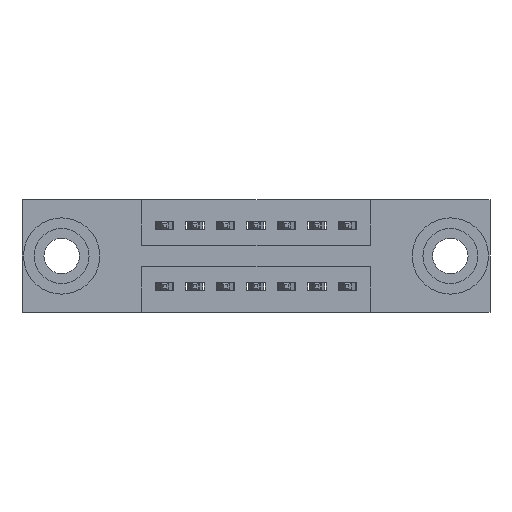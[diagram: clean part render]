
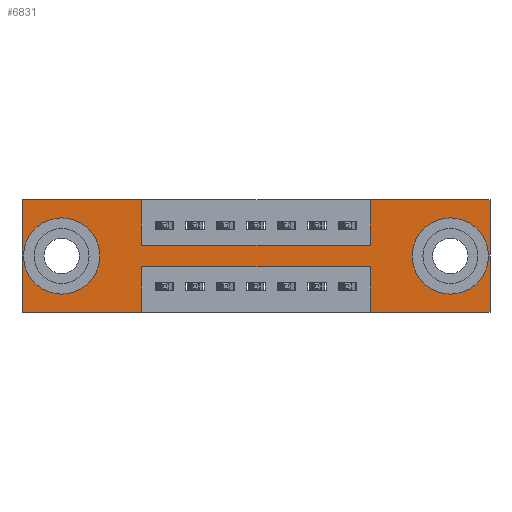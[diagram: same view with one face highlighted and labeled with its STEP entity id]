
A CAD part, front view. The second image highlights one B-rep face of the part: STEP entity #6831.
In plain terms, the highlighted planar face has unit normal (0, -1, 0).
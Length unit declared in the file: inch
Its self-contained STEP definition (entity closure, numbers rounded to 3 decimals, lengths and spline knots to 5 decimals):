
#35 = DIRECTION ( 'NONE',  ( 1., 0., 0. ) ) ;
#153 = CIRCLE ( 'NONE', #6250, 0.078 ) ;
#190 = ORIENTED_EDGE ( 'NONE', *, *, #2912, .T. ) ;
#196 = VERTEX_POINT ( 'NONE', #5397 ) ;
#292 = DIRECTION ( 'NONE',  ( 0., 0., 1. ) ) ;
#322 = ORIENTED_EDGE ( 'NONE', *, *, #9710, .F. ) ;
#339 = ORIENTED_EDGE ( 'NONE', *, *, #6166, .F. ) ;
#712 = LINE ( 'NONE', #8109, #2543 ) ;
#912 = EDGE_LOOP ( 'NONE', ( #339, #1281, #2503, #10819, #2200, #2642, #5281, #9050, #322, #3176, #4669, #4820 ) ) ;
#993 = VECTOR ( 'NONE', #8894, 39.37008 ) ;
#1029 = DIRECTION ( 'NONE',  ( 0., 1., 0. ) ) ;
#1041 = CARTESIAN_POINT ( 'NONE',  ( 1.405, 0., -0.107 ) ) ;
#1169 = DIRECTION ( 'NONE',  ( 0., 1., 0. ) ) ;
#1196 = DIRECTION ( 'NONE',  ( 0., -1., 0. ) ) ;
#1241 = DIRECTION ( 'NONE',  ( -1., 0., 0. ) ) ;
#1276 = CARTESIAN_POINT ( 'NONE',  ( 0., 0., 0. ) ) ;
#1281 = ORIENTED_EDGE ( 'NONE', *, *, #8150, .F. ) ;
#1425 = CARTESIAN_POINT ( 'NONE',  ( 0., 0., 0. ) ) ;
#1426 = CARTESIAN_POINT ( 'NONE',  ( 0.13, 0., -0.107 ) ) ;
#1484 = CARTESIAN_POINT ( 'NONE',  ( 1.1425, 0., -0.15 ) ) ;
#1490 = VECTOR ( 'NONE', #9265, 39.37008 ) ;
#1524 = CARTESIAN_POINT ( 'NONE',  ( 1.535, 0., 0. ) ) ;
#1543 = VECTOR ( 'NONE', #2429, 39.37008 ) ;
#1681 = DIRECTION ( 'NONE',  ( 0., 0., -1. ) ) ;
#1714 = DIRECTION ( 'NONE',  ( 0., 1., 0. ) ) ;
#1771 = LINE ( 'NONE', #2597, #1490 ) ;
#1783 = CARTESIAN_POINT ( 'NONE',  ( 1.405, 0., -0.185 ) ) ;
#1834 = VECTOR ( 'NONE', #7708, 39.37008 ) ;
#1903 = ORIENTED_EDGE ( 'NONE', *, *, #5004, .T. ) ;
#1976 = CARTESIAN_POINT ( 'NONE',  ( 0.13, 0., -0.263 ) ) ;
#2084 = FACE_BOUND ( 'NONE', #3840, .T. ) ;
#2121 = VERTEX_POINT ( 'NONE', #4787 ) ;
#2133 = CARTESIAN_POINT ( 'NONE',  ( 0., 0., -0.37 ) ) ;
#2169 = LINE ( 'NONE', #1425, #6464 ) ;
#2200 = ORIENTED_EDGE ( 'NONE', *, *, #6465, .F. ) ;
#2245 = VECTOR ( 'NONE', #5411, 39.37008 ) ;
#2429 = DIRECTION ( 'NONE',  ( 0., 0., -1. ) ) ;
#2431 = VERTEX_POINT ( 'NONE', #1426 ) ;
#2474 = VERTEX_POINT ( 'NONE', #10308 ) ;
#2503 = ORIENTED_EDGE ( 'NONE', *, *, #5922, .F. ) ;
#2543 = VECTOR ( 'NONE', #3100, 39.37008 ) ;
#2597 = CARTESIAN_POINT ( 'NONE',  ( 0.3925, 0., 0. ) ) ;
#2642 = ORIENTED_EDGE ( 'NONE', *, *, #5059, .F. ) ;
#2845 = LINE ( 'NONE', #5032, #5088 ) ;
#2912 = EDGE_CURVE ( 'NONE', #6247, #6154, #6344, .T. ) ;
#3100 = DIRECTION ( 'NONE',  ( 1., 0., 0. ) ) ;
#3105 = EDGE_CURVE ( 'NONE', #8250, #6004, #2169, .T. ) ;
#3176 = ORIENTED_EDGE ( 'NONE', *, *, #3105, .F. ) ;
#3223 = LINE ( 'NONE', #7791, #9541 ) ;
#3261 = VECTOR ( 'NONE', #9844, 39.37008 ) ;
#3314 = CARTESIAN_POINT ( 'NONE',  ( 1.1425, 0., -0.37 ) ) ;
#3840 = EDGE_LOOP ( 'NONE', ( #8541, #190 ) ) ;
#3850 = ORIENTED_EDGE ( 'NONE', *, *, #4265, .T. ) ;
#3860 = VECTOR ( 'NONE', #1241, 39.37008 ) ;
#4164 = CARTESIAN_POINT ( 'NONE',  ( 0.3925, 0., -0.15 ) ) ;
#4219 = EDGE_CURVE ( 'NONE', #5334, #4577, #2845, .T. ) ;
#4265 = EDGE_CURVE ( 'NONE', #8760, #2431, #153, .T. ) ;
#4519 = EDGE_CURVE ( 'NONE', #196, #8250, #7235, .T. ) ;
#4528 = LINE ( 'NONE', #4578, #9403 ) ;
#4534 = VERTEX_POINT ( 'NONE', #1484 ) ;
#4577 = VERTEX_POINT ( 'NONE', #3314 ) ;
#4578 = CARTESIAN_POINT ( 'NONE',  ( 0.3925, 0., -0.22 ) ) ;
#4655 = FACE_OUTER_BOUND ( 'NONE', #912, .T. ) ;
#4669 = ORIENTED_EDGE ( 'NONE', *, *, #4519, .F. ) ;
#4693 = CARTESIAN_POINT ( 'NONE',  ( 0.3925, 0., -0.22 ) ) ;
#4712 = CARTESIAN_POINT ( 'NONE',  ( 1.405, 0., -0.263 ) ) ;
#4787 = CARTESIAN_POINT ( 'NONE',  ( 1.535, 0., 0. ) ) ;
#4803 = LINE ( 'NONE', #6277, #2245 ) ;
#4820 = ORIENTED_EDGE ( 'NONE', *, *, #8890, .F. ) ;
#4956 = CIRCLE ( 'NONE', #7176, 0.078 ) ;
#5004 = EDGE_CURVE ( 'NONE', #2431, #8760, #4956, .T. ) ;
#5032 = CARTESIAN_POINT ( 'NONE',  ( 0., 0., -0.37 ) ) ;
#5059 = EDGE_CURVE ( 'NONE', #5090, #2121, #5572, .T. ) ;
#5088 = VECTOR ( 'NONE', #7942, 39.37008 ) ;
#5090 = VERTEX_POINT ( 'NONE', #9714 ) ;
#5281 = ORIENTED_EDGE ( 'NONE', *, *, #7440, .F. ) ;
#5296 = AXIS2_PLACEMENT_3D ( 'NONE', #6232, #1029, #7084 ) ;
#5334 = VERTEX_POINT ( 'NONE', #7845 ) ;
#5379 = DIRECTION ( 'NONE',  ( -1., 0., 0. ) ) ;
#5391 = CIRCLE ( 'NONE', #5296, 0.078 ) ;
#5397 = CARTESIAN_POINT ( 'NONE',  ( 0., 0., -0.37 ) ) ;
#5411 = DIRECTION ( 'NONE',  ( 0., 0., -1. ) ) ;
#5503 = DIRECTION ( 'NONE',  ( 0., 1., 0. ) ) ;
#5572 = LINE ( 'NONE', #1276, #993 ) ;
#5612 = EDGE_CURVE ( 'NONE', #8415, #4534, #712, .T. ) ;
#5922 = EDGE_CURVE ( 'NONE', #4577, #9687, #6406, .T. ) ;
#6004 = VERTEX_POINT ( 'NONE', #7778 ) ;
#6134 = LINE ( 'NONE', #1524, #1543 ) ;
#6154 = VERTEX_POINT ( 'NONE', #1041 ) ;
#6166 = EDGE_CURVE ( 'NONE', #9340, #2474, #4803, .T. ) ;
#6232 = CARTESIAN_POINT ( 'NONE',  ( 1.405, 0., -0.185 ) ) ;
#6247 = VERTEX_POINT ( 'NONE', #4712 ) ;
#6250 = AXIS2_PLACEMENT_3D ( 'NONE', #6354, #1169, #7197 ) ;
#6277 = CARTESIAN_POINT ( 'NONE',  ( 0.3925, 0., -0.37 ) ) ;
#6342 = CARTESIAN_POINT ( 'NONE',  ( 0., 0., -0.37 ) ) ;
#6344 = CIRCLE ( 'NONE', #7311, 0.078 ) ;
#6354 = CARTESIAN_POINT ( 'NONE',  ( 0.13, 0., -0.185 ) ) ;
#6381 = PLANE ( 'NONE',  #8669 ) ;
#6406 = LINE ( 'NONE', #9258, #1834 ) ;
#6464 = VECTOR ( 'NONE', #35, 39.37008 ) ;
#6465 = EDGE_CURVE ( 'NONE', #2121, #5334, #6134, .T. ) ;
#6639 = LINE ( 'NONE', #2133, #3860 ) ;
#6831 = ADVANCED_FACE ( 'NONE', ( #2084, #8816, #4655 ), #6381, .T. ) ;
#6997 = DIRECTION ( 'NONE',  ( 0., 0., 1. ) ) ;
#7084 = DIRECTION ( 'NONE',  ( 0., 0., -1. ) ) ;
#7176 = AXIS2_PLACEMENT_3D ( 'NONE', #10390, #5503, #292 ) ;
#7197 = DIRECTION ( 'NONE',  ( 0., 0., 1. ) ) ;
#7229 = DIRECTION ( 'NONE',  ( 0., 0., -1. ) ) ;
#7235 = LINE ( 'NONE', #8238, #3261 ) ;
#7311 = AXIS2_PLACEMENT_3D ( 'NONE', #1783, #1714, #1681 ) ;
#7440 = EDGE_CURVE ( 'NONE', #4534, #5090, #3223, .T. ) ;
#7708 = DIRECTION ( 'NONE',  ( 0., 0., 1. ) ) ;
#7778 = CARTESIAN_POINT ( 'NONE',  ( 0.3925, 0., 0. ) ) ;
#7791 = CARTESIAN_POINT ( 'NONE',  ( 1.1425, 0., 0. ) ) ;
#7845 = CARTESIAN_POINT ( 'NONE',  ( 1.535, 0., -0.37 ) ) ;
#7942 = DIRECTION ( 'NONE',  ( -1., 0., 0. ) ) ;
#8109 = CARTESIAN_POINT ( 'NONE',  ( 0.3925, 0., -0.15 ) ) ;
#8150 = EDGE_CURVE ( 'NONE', #9687, #9340, #4528, .T. ) ;
#8238 = CARTESIAN_POINT ( 'NONE',  ( 0., 0., 0. ) ) ;
#8250 = VERTEX_POINT ( 'NONE', #8789 ) ;
#8415 = VERTEX_POINT ( 'NONE', #4164 ) ;
#8463 = CARTESIAN_POINT ( 'NONE',  ( 1.1425, 0., -0.22 ) ) ;
#8541 = ORIENTED_EDGE ( 'NONE', *, *, #8720, .T. ) ;
#8669 = AXIS2_PLACEMENT_3D ( 'NONE', #6342, #1196, #7229 ) ;
#8720 = EDGE_CURVE ( 'NONE', #6154, #6247, #5391, .T. ) ;
#8760 = VERTEX_POINT ( 'NONE', #1976 ) ;
#8789 = CARTESIAN_POINT ( 'NONE',  ( 0., 0., 0. ) ) ;
#8816 = FACE_BOUND ( 'NONE', #8982, .T. ) ;
#8890 = EDGE_CURVE ( 'NONE', #2474, #196, #6639, .T. ) ;
#8894 = DIRECTION ( 'NONE',  ( 1., 0., 0. ) ) ;
#8982 = EDGE_LOOP ( 'NONE', ( #1903, #3850 ) ) ;
#9050 = ORIENTED_EDGE ( 'NONE', *, *, #5612, .F. ) ;
#9258 = CARTESIAN_POINT ( 'NONE',  ( 1.1425, 0., -0.37 ) ) ;
#9265 = DIRECTION ( 'NONE',  ( 0., 0., -1. ) ) ;
#9340 = VERTEX_POINT ( 'NONE', #4693 ) ;
#9403 = VECTOR ( 'NONE', #5379, 39.37008 ) ;
#9541 = VECTOR ( 'NONE', #6997, 39.37008 ) ;
#9687 = VERTEX_POINT ( 'NONE', #8463 ) ;
#9710 = EDGE_CURVE ( 'NONE', #6004, #8415, #1771, .T. ) ;
#9714 = CARTESIAN_POINT ( 'NONE',  ( 1.1425, 0., 0. ) ) ;
#9844 = DIRECTION ( 'NONE',  ( 0., 0., 1. ) ) ;
#10308 = CARTESIAN_POINT ( 'NONE',  ( 0.3925, 0., -0.37 ) ) ;
#10390 = CARTESIAN_POINT ( 'NONE',  ( 0.13, 0., -0.185 ) ) ;
#10819 = ORIENTED_EDGE ( 'NONE', *, *, #4219, .F. ) ;
